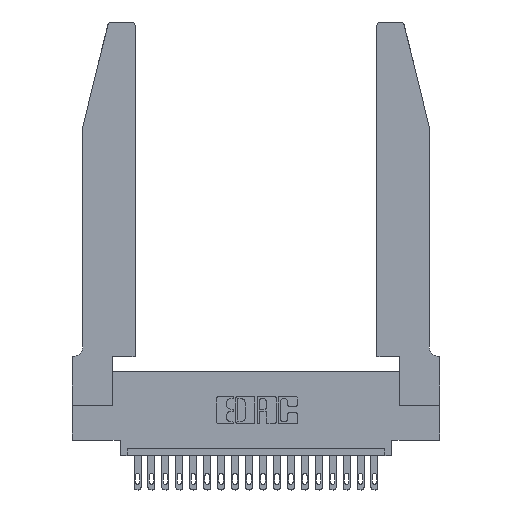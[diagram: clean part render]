
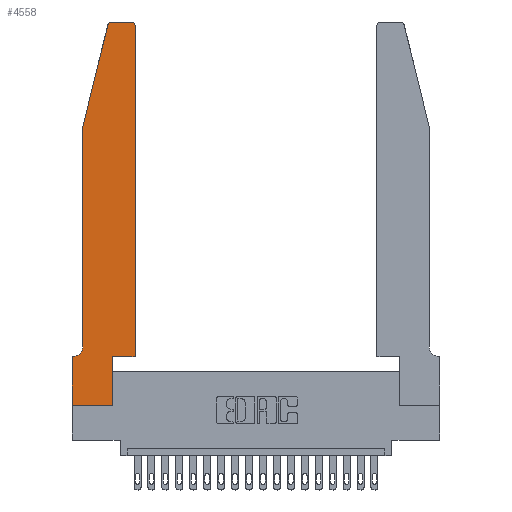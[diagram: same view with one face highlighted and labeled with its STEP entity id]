
A CAD part, top view. The second image highlights one B-rep face of the part: STEP entity #4558.
In plain terms, the highlighted planar face has unit normal (0, 0, 1).
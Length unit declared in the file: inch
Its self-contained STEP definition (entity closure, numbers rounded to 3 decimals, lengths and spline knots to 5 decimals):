
#310 = CARTESIAN_POINT ( 'NONE',  ( 0., 0.35, 0.37 ) ) ;
#737 = DIRECTION ( 'NONE',  ( 0., 0., 1. ) ) ;
#883 = VECTOR ( 'NONE', #1334, 39.37008 ) ;
#1211 = CARTESIAN_POINT ( 'NONE',  ( 0.4505, 2.72, 0.37 ) ) ;
#1334 = DIRECTION ( 'NONE',  ( 0., -1., 0. ) ) ;
#1411 = CARTESIAN_POINT ( 'NONE',  ( 0.0755, 2., 0.37 ) ) ;
#1498 = CARTESIAN_POINT ( 'NONE',  ( 0.284, 2.75, 0.37 ) ) ;
#1727 = EDGE_CURVE ( 'NONE', #13619, #18205, #5067, .T. ) ;
#2607 = FACE_OUTER_BOUND ( 'NONE', #4871, .T. ) ;
#3372 = CARTESIAN_POINT ( 'NONE',  ( 0.4505, 0.35, 0.37 ) ) ;
#3539 = CARTESIAN_POINT ( 'NONE',  ( 0., 0.35, 0.37 ) ) ;
#3984 = EDGE_CURVE ( 'NONE', #9602, #10801, #20635, .T. ) ;
#4545 = DIRECTION ( 'NONE',  ( 0., 0., -1. ) ) ;
#4557 = CARTESIAN_POINT ( 'NONE',  ( 0., 0., 0.37 ) ) ;
#4558 = ADVANCED_FACE ( 'NONE', ( #2607 ), #16849, .T. ) ;
#4780 = ORIENTED_EDGE ( 'NONE', *, *, #1727, .T. ) ;
#4871 = EDGE_LOOP ( 'NONE', ( #7657, #15634, #7128, #4780, #21183, #10075, #10295, #15310, #19592, #9933, #13368, #16733 ) ) ;
#4916 = LINE ( 'NONE', #14061, #7801 ) ;
#4963 = CARTESIAN_POINT ( 'NONE',  ( 0.284, 2.72, 0.37 ) ) ;
#5006 = EDGE_CURVE ( 'NONE', #18205, #11165, #10899, .T. ) ;
#5067 = LINE ( 'NONE', #10389, #13098 ) ;
#5473 = CARTESIAN_POINT ( 'NONE',  ( 0.4505, 0.35, 0.37 ) ) ;
#5814 = VERTEX_POINT ( 'NONE', #5473 ) ;
#5902 = AXIS2_PLACEMENT_3D ( 'NONE', #310, #737, #17278 ) ;
#6046 = VECTOR ( 'NONE', #16265, 39.37008 ) ;
#6201 = VECTOR ( 'NONE', #10051, 39.37008 ) ;
#6354 = VERTEX_POINT ( 'NONE', #20148 ) ;
#6395 = LINE ( 'NONE', #16183, #883 ) ;
#6691 = CIRCLE ( 'NONE', #8650, 0.03 ) ;
#7128 = ORIENTED_EDGE ( 'NONE', *, *, #14988, .T. ) ;
#7216 = DIRECTION ( 'NONE',  ( 0., 0., 1. ) ) ;
#7580 = EDGE_CURVE ( 'NONE', #18224, #13104, #6395, .T. ) ;
#7643 = CARTESIAN_POINT ( 'NONE',  ( 0.0755, 2., 0.37 ) ) ;
#7657 = ORIENTED_EDGE ( 'NONE', *, *, #16025, .T. ) ;
#7801 = VECTOR ( 'NONE', #20955, 39.37008 ) ;
#8080 = CARTESIAN_POINT ( 'NONE',  ( 0., 0., 0.37 ) ) ;
#8455 = CARTESIAN_POINT ( 'NONE',  ( 0.2865, 0.35, 0.37 ) ) ;
#8495 = VECTOR ( 'NONE', #12976, 39.37008 ) ;
#8603 = DIRECTION ( 'NONE',  ( -1., 0., 0. ) ) ;
#8650 = AXIS2_PLACEMENT_3D ( 'NONE', #15772, #7216, #8892 ) ;
#8892 = DIRECTION ( 'NONE',  ( 1., 0., 0. ) ) ;
#8959 = CARTESIAN_POINT ( 'NONE',  ( 0.0055, 0.35, 0.37 ) ) ;
#9036 = DIRECTION ( 'NONE',  ( 0., 1., 0. ) ) ;
#9283 = VECTOR ( 'NONE', #9036, 39.37008 ) ;
#9602 = VERTEX_POINT ( 'NONE', #1498 ) ;
#9678 = CARTESIAN_POINT ( 'NONE',  ( 0.4505, 0.35, 0.37 ) ) ;
#9767 = CARTESIAN_POINT ( 'NONE',  ( 0.25487, 2.72718, 0.37 ) ) ;
#9933 = ORIENTED_EDGE ( 'NONE', *, *, #20182, .T. ) ;
#10051 = DIRECTION ( 'NONE',  ( 1., 0., 0. ) ) ;
#10075 = ORIENTED_EDGE ( 'NONE', *, *, #17553, .T. ) ;
#10219 = CARTESIAN_POINT ( 'NONE',  ( 0.0755, 0.42, 0.37 ) ) ;
#10295 = ORIENTED_EDGE ( 'NONE', *, *, #7580, .T. ) ;
#10389 = CARTESIAN_POINT ( 'NONE',  ( 0.0755, 2., 0.37 ) ) ;
#10606 = DIRECTION ( 'NONE',  ( 0., -1., 0. ) ) ;
#10682 = VERTEX_POINT ( 'NONE', #1211 ) ;
#10801 = VERTEX_POINT ( 'NONE', #9767 ) ;
#10877 = AXIS2_PLACEMENT_3D ( 'NONE', #4963, #19964, #11496 ) ;
#10899 = CIRCLE ( 'NONE', #19388, 0.07 ) ;
#11165 = VERTEX_POINT ( 'NONE', #8959 ) ;
#11496 = DIRECTION ( 'NONE',  ( 1., 0., 0. ) ) ;
#11623 = CARTESIAN_POINT ( 'NONE',  ( 0.0755, 0.35, 0.37 ) ) ;
#12665 = VERTEX_POINT ( 'NONE', #8455 ) ;
#12976 = DIRECTION ( 'NONE',  ( 0., 1., 0. ) ) ;
#13098 = VECTOR ( 'NONE', #10606, 39.37008 ) ;
#13104 = VERTEX_POINT ( 'NONE', #8080 ) ;
#13368 = ORIENTED_EDGE ( 'NONE', *, *, #17882, .T. ) ;
#13575 = EDGE_CURVE ( 'NONE', #13104, #19017, #19552, .T. ) ;
#13619 = VERTEX_POINT ( 'NONE', #1411 ) ;
#14061 = CARTESIAN_POINT ( 'NONE',  ( 0.2605, 2.75, 0.37 ) ) ;
#14280 = DIRECTION ( 'NONE',  ( -0.239, -0.971, 0. ) ) ;
#14435 = LINE ( 'NONE', #18760, #9283 ) ;
#14476 = CARTESIAN_POINT ( 'NONE',  ( 0.0055, 0.42, 0.37 ) ) ;
#14654 = CARTESIAN_POINT ( 'NONE',  ( 0.2865, 0., 0.37 ) ) ;
#14975 = VECTOR ( 'NONE', #8603, 39.37008 ) ;
#14988 = EDGE_CURVE ( 'NONE', #10801, #13619, #16931, .T. ) ;
#15310 = ORIENTED_EDGE ( 'NONE', *, *, #13575, .T. ) ;
#15634 = ORIENTED_EDGE ( 'NONE', *, *, #3984, .T. ) ;
#15772 = CARTESIAN_POINT ( 'NONE',  ( 0.4205, 2.72, 0.37 ) ) ;
#16025 = EDGE_CURVE ( 'NONE', #6354, #9602, #4916, .T. ) ;
#16177 = DIRECTION ( 'NONE',  ( -1., 0., 0. ) ) ;
#16183 = CARTESIAN_POINT ( 'NONE',  ( 0., 0., 0.37 ) ) ;
#16265 = DIRECTION ( 'NONE',  ( 1., 0., 0. ) ) ;
#16733 = ORIENTED_EDGE ( 'NONE', *, *, #20470, .T. ) ;
#16849 = PLANE ( 'NONE',  #5902 ) ;
#16931 = LINE ( 'NONE', #7643, #18238 ) ;
#17278 = DIRECTION ( 'NONE',  ( 1., 0., 0. ) ) ;
#17553 = EDGE_CURVE ( 'NONE', #11165, #18224, #19422, .T. ) ;
#17644 = LINE ( 'NONE', #3372, #6201 ) ;
#17714 = EDGE_CURVE ( 'NONE', #19017, #12665, #14435, .T. ) ;
#17882 = EDGE_CURVE ( 'NONE', #5814, #10682, #19415, .T. ) ;
#18205 = VERTEX_POINT ( 'NONE', #10219 ) ;
#18224 = VERTEX_POINT ( 'NONE', #3539 ) ;
#18238 = VECTOR ( 'NONE', #14280, 39.37008 ) ;
#18760 = CARTESIAN_POINT ( 'NONE',  ( 0.2865, 0.35, 0.37 ) ) ;
#19017 = VERTEX_POINT ( 'NONE', #14654 ) ;
#19388 = AXIS2_PLACEMENT_3D ( 'NONE', #14476, #4545, #16177 ) ;
#19415 = LINE ( 'NONE', #9678, #8495 ) ;
#19422 = LINE ( 'NONE', #11623, #14975 ) ;
#19552 = LINE ( 'NONE', #4557, #6046 ) ;
#19592 = ORIENTED_EDGE ( 'NONE', *, *, #17714, .T. ) ;
#19964 = DIRECTION ( 'NONE',  ( 0., 0., 1. ) ) ;
#20148 = CARTESIAN_POINT ( 'NONE',  ( 0.4205, 2.75, 0.37 ) ) ;
#20182 = EDGE_CURVE ( 'NONE', #12665, #5814, #17644, .T. ) ;
#20470 = EDGE_CURVE ( 'NONE', #10682, #6354, #6691, .T. ) ;
#20635 = CIRCLE ( 'NONE', #10877, 0.03 ) ;
#20955 = DIRECTION ( 'NONE',  ( -1., 0., 0. ) ) ;
#21183 = ORIENTED_EDGE ( 'NONE', *, *, #5006, .T. ) ;
